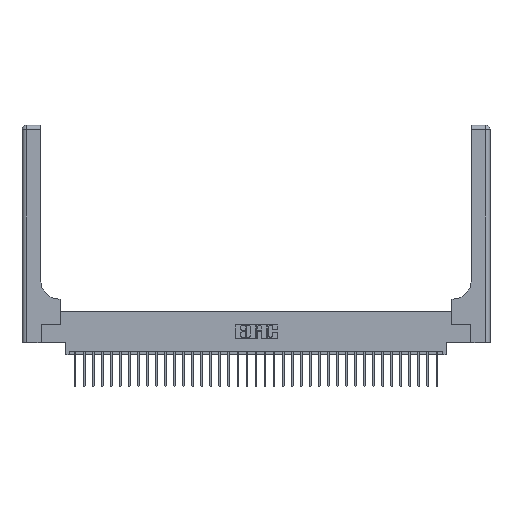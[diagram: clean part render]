
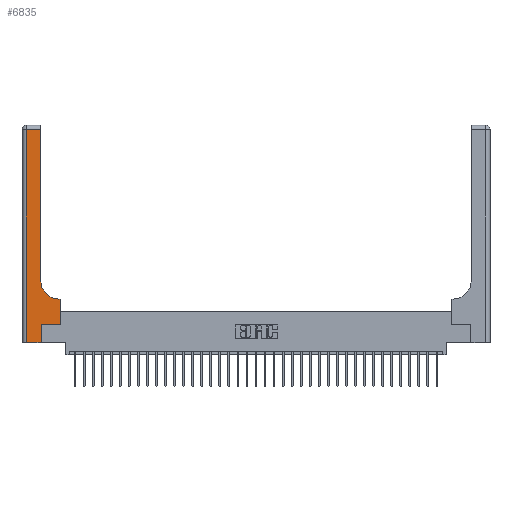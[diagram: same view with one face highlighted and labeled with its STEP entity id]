
A CAD part, top view. The second image highlights one B-rep face of the part: STEP entity #6835.
In plain terms, the highlighted planar face has unit normal (0, 0, 1).
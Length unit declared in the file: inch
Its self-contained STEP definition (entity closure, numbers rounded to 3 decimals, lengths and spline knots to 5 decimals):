
#70 = EDGE_CURVE ( 'NONE', #12508, #29380, #24568, .T. ) ;
#1171 = AXIS2_PLACEMENT_3D ( 'NONE', #3844, #21234, #6328 ) ;
#1327 = ORIENTED_EDGE ( 'NONE', *, *, #3311, .T. ) ;
#1712 = VERTEX_POINT ( 'NONE', #12001 ) ;
#2240 = ORIENTED_EDGE ( 'NONE', *, *, #23991, .T. ) ;
#2671 = CARTESIAN_POINT ( 'NONE',  ( 0., 3., 0.37 ) ) ;
#2682 = CARTESIAN_POINT ( 'NONE',  ( 0.06, 0., 0.37 ) ) ;
#2691 = VECTOR ( 'NONE', #21150, 39.37008 ) ;
#3274 = DIRECTION ( 'NONE',  ( 0., -1., 0. ) ) ;
#3311 = EDGE_CURVE ( 'NONE', #9208, #7252, #19280, .T. ) ;
#3749 = CARTESIAN_POINT ( 'NONE',  ( 0.26, 3., 0.37 ) ) ;
#3844 = CARTESIAN_POINT ( 'NONE',  ( 0.51, 0.85, 0.37 ) ) ;
#4673 = ORIENTED_EDGE ( 'NONE', *, *, #21432, .T. ) ;
#4804 = VERTEX_POINT ( 'NONE', #2682 ) ;
#4901 = DIRECTION ( 'NONE',  ( 0., 1., 0. ) ) ;
#6328 = DIRECTION ( 'NONE',  ( 1., 0., 0. ) ) ;
#6612 = FACE_OUTER_BOUND ( 'NONE', #25904, .T. ) ;
#6835 = ADVANCED_FACE ( 'NONE', ( #6612 ), #27503, .F. ) ;
#6958 = EDGE_CURVE ( 'NONE', #29380, #15507, #22581, .T. ) ;
#7252 = VERTEX_POINT ( 'NONE', #31819 ) ;
#7693 = DIRECTION ( 'NONE',  ( 0., 0., -1. ) ) ;
#8049 = LINE ( 'NONE', #24941, #26371 ) ;
#8237 = CARTESIAN_POINT ( 'NONE',  ( 0., 2.94, 0.37 ) ) ;
#8892 = VECTOR ( 'NONE', #13059, 39.37008 ) ;
#9008 = DIRECTION ( 'NONE',  ( 1., 0., 0. ) ) ;
#9208 = VERTEX_POINT ( 'NONE', #22774 ) ;
#9919 = CARTESIAN_POINT ( 'NONE',  ( 0.265, 0., 0.37 ) ) ;
#10559 = CARTESIAN_POINT ( 'NONE',  ( 0.528, 0.25, 0.37 ) ) ;
#12001 = CARTESIAN_POINT ( 'NONE',  ( 0.528, 0.6, 0.37 ) ) ;
#12215 = ORIENTED_EDGE ( 'NONE', *, *, #70, .T. ) ;
#12508 = VERTEX_POINT ( 'NONE', #28278 ) ;
#12597 = EDGE_CURVE ( 'NONE', #26253, #9208, #15134, .T. ) ;
#13059 = DIRECTION ( 'NONE',  ( 0., 1., 0. ) ) ;
#13860 = CARTESIAN_POINT ( 'NONE',  ( 0.26, 0.85, 0.37 ) ) ;
#13908 = CIRCLE ( 'NONE', #1171, 0.25 ) ;
#13956 = EDGE_CURVE ( 'NONE', #18292, #26253, #13908, .T. ) ;
#14008 = CARTESIAN_POINT ( 'NONE',  ( 0., 0., 0.37 ) ) ;
#14691 = EDGE_CURVE ( 'NONE', #4804, #12508, #24505, .T. ) ;
#14815 = ORIENTED_EDGE ( 'NONE', *, *, #12597, .T. ) ;
#15134 = LINE ( 'NONE', #3749, #2691 ) ;
#15507 = VERTEX_POINT ( 'NONE', #17199 ) ;
#15936 = VECTOR ( 'NONE', #25534, 39.37008 ) ;
#17141 = ORIENTED_EDGE ( 'NONE', *, *, #13956, .T. ) ;
#17199 = CARTESIAN_POINT ( 'NONE',  ( 0.528, 0.25, 0.37 ) ) ;
#17892 = ORIENTED_EDGE ( 'NONE', *, *, #22445, .T. ) ;
#17908 = VECTOR ( 'NONE', #4901, 39.37008 ) ;
#17956 = CARTESIAN_POINT ( 'NONE',  ( 0.51, 0.6, 0.37 ) ) ;
#18292 = VERTEX_POINT ( 'NONE', #17956 ) ;
#18505 = VECTOR ( 'NONE', #28199, 39.37008 ) ;
#19118 = CARTESIAN_POINT ( 'NONE',  ( 0.265, 0.25, 0.37 ) ) ;
#19280 = LINE ( 'NONE', #8237, #18505 ) ;
#20696 = CARTESIAN_POINT ( 'NONE',  ( 0.06, 3., 0.37 ) ) ;
#21150 = DIRECTION ( 'NONE',  ( 0., 1., 0. ) ) ;
#21234 = DIRECTION ( 'NONE',  ( 0., 0., -1. ) ) ;
#21432 = EDGE_CURVE ( 'NONE', #15507, #1712, #22134, .T. ) ;
#22134 = LINE ( 'NONE', #10559, #8892 ) ;
#22445 = EDGE_CURVE ( 'NONE', #1712, #18292, #8049, .T. ) ;
#22581 = LINE ( 'NONE', #27953, #15936 ) ;
#22774 = CARTESIAN_POINT ( 'NONE',  ( 0.26, 2.94, 0.37 ) ) ;
#23991 = EDGE_CURVE ( 'NONE', #7252, #4804, #30151, .T. ) ;
#24273 = ORIENTED_EDGE ( 'NONE', *, *, #14691, .T. ) ;
#24505 = LINE ( 'NONE', #14008, #28048 ) ;
#24568 = LINE ( 'NONE', #9919, #17908 ) ;
#24941 = CARTESIAN_POINT ( 'NONE',  ( 0.26, 0.6, 0.37 ) ) ;
#25096 = DIRECTION ( 'NONE',  ( -1., 0., 0. ) ) ;
#25534 = DIRECTION ( 'NONE',  ( 1., 0., 0. ) ) ;
#25885 = AXIS2_PLACEMENT_3D ( 'NONE', #2671, #7693, #25096 ) ;
#25904 = EDGE_LOOP ( 'NONE', ( #14815, #1327, #2240, #24273, #12215, #29049, #4673, #17892, #17141 ) ) ;
#26253 = VERTEX_POINT ( 'NONE', #13860 ) ;
#26371 = VECTOR ( 'NONE', #27445, 39.37008 ) ;
#27445 = DIRECTION ( 'NONE',  ( -1., 0., 0. ) ) ;
#27503 = PLANE ( 'NONE',  #25885 ) ;
#27953 = CARTESIAN_POINT ( 'NONE',  ( 0.265, 0.25, 0.37 ) ) ;
#28048 = VECTOR ( 'NONE', #9008, 39.37008 ) ;
#28199 = DIRECTION ( 'NONE',  ( -1., 0., 0. ) ) ;
#28278 = CARTESIAN_POINT ( 'NONE',  ( 0.265, 0., 0.37 ) ) ;
#29049 = ORIENTED_EDGE ( 'NONE', *, *, #6958, .T. ) ;
#29359 = VECTOR ( 'NONE', #3274, 39.37008 ) ;
#29380 = VERTEX_POINT ( 'NONE', #19118 ) ;
#30151 = LINE ( 'NONE', #20696, #29359 ) ;
#31819 = CARTESIAN_POINT ( 'NONE',  ( 0.06, 2.94, 0.37 ) ) ;
